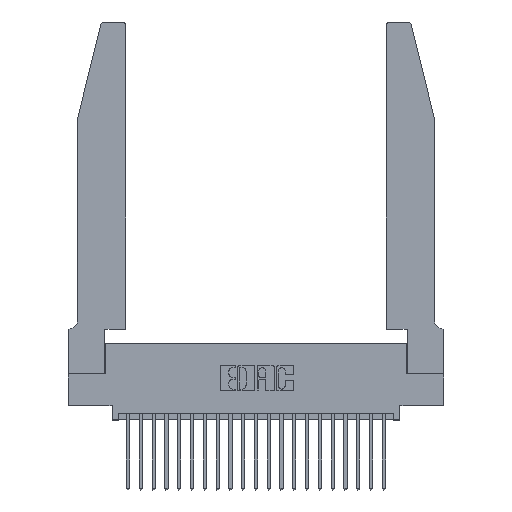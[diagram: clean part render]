
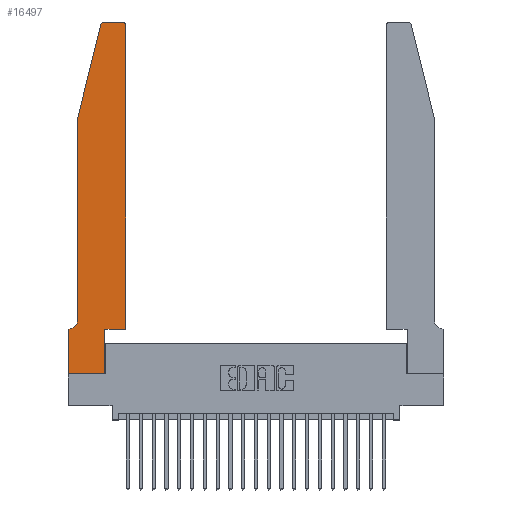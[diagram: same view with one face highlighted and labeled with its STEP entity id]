
A CAD part, top view. The second image highlights one B-rep face of the part: STEP entity #16497.
In plain terms, the highlighted planar face has unit normal (0, 0, 1).
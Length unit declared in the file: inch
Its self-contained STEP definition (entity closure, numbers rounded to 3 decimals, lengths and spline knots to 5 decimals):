
#417 = CIRCLE ( 'NONE', #15618, 0.07 ) ;
#516 = DIRECTION ( 'NONE',  ( 0., -1., 0. ) ) ;
#763 = ORIENTED_EDGE ( 'NONE', *, *, #9248, .T. ) ;
#764 = VECTOR ( 'NONE', #19577, 39.37008 ) ;
#982 = DIRECTION ( 'NONE',  ( 0., 1., 0. ) ) ;
#1370 = DIRECTION ( 'NONE',  ( -1., 0., 0. ) ) ;
#1402 = VECTOR ( 'NONE', #516, 39.37008 ) ;
#1412 = VERTEX_POINT ( 'NONE', #19674 ) ;
#1561 = VERTEX_POINT ( 'NONE', #11043 ) ;
#1594 = VERTEX_POINT ( 'NONE', #15425 ) ;
#1689 = VERTEX_POINT ( 'NONE', #3669 ) ;
#1705 = DIRECTION ( 'NONE',  ( 0., 0., 1. ) ) ;
#1916 = CARTESIAN_POINT ( 'NONE',  ( 0.0755, 2., 0.37 ) ) ;
#2494 = DIRECTION ( 'NONE',  ( 0., -1., 0. ) ) ;
#3249 = VERTEX_POINT ( 'NONE', #17881 ) ;
#3274 = DIRECTION ( 'NONE',  ( 0., 0., 1. ) ) ;
#3669 = CARTESIAN_POINT ( 'NONE',  ( 0.2865, 0., 0.37 ) ) ;
#3691 = VECTOR ( 'NONE', #982, 39.37008 ) ;
#3705 = VERTEX_POINT ( 'NONE', #4144 ) ;
#4137 = CARTESIAN_POINT ( 'NONE',  ( 0.2865, 0.35, 0.37 ) ) ;
#4144 = CARTESIAN_POINT ( 'NONE',  ( 0.284, 2.75, 0.37 ) ) ;
#4436 = AXIS2_PLACEMENT_3D ( 'NONE', #14583, #3274, #16380 ) ;
#4560 = CARTESIAN_POINT ( 'NONE',  ( 0.4205, 2.72, 0.37 ) ) ;
#4660 = CIRCLE ( 'NONE', #8988, 0.03 ) ;
#4784 = CARTESIAN_POINT ( 'NONE',  ( 0.4505, 0.35, 0.37 ) ) ;
#4839 = ORIENTED_EDGE ( 'NONE', *, *, #18056, .T. ) ;
#5339 = CARTESIAN_POINT ( 'NONE',  ( 0.2605, 2.75, 0.37 ) ) ;
#5398 = CARTESIAN_POINT ( 'NONE',  ( 0., 0.35, 0.37 ) ) ;
#5412 = EDGE_CURVE ( 'NONE', #1689, #17257, #23343, .T. ) ;
#5982 = CARTESIAN_POINT ( 'NONE',  ( 0.0755, 0.42, 0.37 ) ) ;
#6027 = LINE ( 'NONE', #19297, #1402 ) ;
#6496 = DIRECTION ( 'NONE',  ( 1., 0., 0. ) ) ;
#6662 = ORIENTED_EDGE ( 'NONE', *, *, #22767, .T. ) ;
#7354 = CARTESIAN_POINT ( 'NONE',  ( 0.25487, 2.72718, 0.37 ) ) ;
#8195 = VECTOR ( 'NONE', #2494, 39.37008 ) ;
#8217 = EDGE_CURVE ( 'NONE', #1594, #16972, #14595, .T. ) ;
#8499 = ORIENTED_EDGE ( 'NONE', *, *, #14826, .T. ) ;
#8736 = VECTOR ( 'NONE', #1370, 39.37008 ) ;
#8988 = AXIS2_PLACEMENT_3D ( 'NONE', #4560, #17552, #6496 ) ;
#9087 = VECTOR ( 'NONE', #19044, 39.37008 ) ;
#9248 = EDGE_CURVE ( 'NONE', #17257, #3249, #18185, .T. ) ;
#9323 = LINE ( 'NONE', #5339, #8736 ) ;
#9379 = PLANE ( 'NONE',  #18551 ) ;
#9465 = ORIENTED_EDGE ( 'NONE', *, *, #9613, .T. ) ;
#9613 = EDGE_CURVE ( 'NONE', #20555, #19728, #10246, .T. ) ;
#9789 = DIRECTION ( 'NONE',  ( 1., 0., 0. ) ) ;
#10006 = CARTESIAN_POINT ( 'NONE',  ( 0.4505, 0.35, 0.37 ) ) ;
#10242 = CARTESIAN_POINT ( 'NONE',  ( 0.0755, 0.35, 0.37 ) ) ;
#10246 = LINE ( 'NONE', #21478, #24086 ) ;
#10759 = ORIENTED_EDGE ( 'NONE', *, *, #22531, .T. ) ;
#11043 = CARTESIAN_POINT ( 'NONE',  ( 0., 0., 0.37 ) ) ;
#11583 = CARTESIAN_POINT ( 'NONE',  ( 0.0055, 0.42, 0.37 ) ) ;
#12852 = FACE_OUTER_BOUND ( 'NONE', #15964, .T. ) ;
#13400 = DIRECTION ( 'NONE',  ( -1., 0., 0. ) ) ;
#13519 = CIRCLE ( 'NONE', #4436, 0.03 ) ;
#13804 = LINE ( 'NONE', #22463, #22829 ) ;
#13898 = EDGE_CURVE ( 'NONE', #3705, #20555, #13519, .T. ) ;
#14163 = DIRECTION ( 'NONE',  ( -0.239, -0.971, 0. ) ) ;
#14305 = ORIENTED_EDGE ( 'NONE', *, *, #5412, .T. ) ;
#14439 = ORIENTED_EDGE ( 'NONE', *, *, #8217, .T. ) ;
#14583 = CARTESIAN_POINT ( 'NONE',  ( 0.284, 2.72, 0.37 ) ) ;
#14595 = LINE ( 'NONE', #10242, #18795 ) ;
#14826 = EDGE_CURVE ( 'NONE', #1561, #1689, #13804, .T. ) ;
#14987 = DIRECTION ( 'NONE',  ( 1., 0., 0. ) ) ;
#15004 = EDGE_CURVE ( 'NONE', #19260, #1412, #4660, .T. ) ;
#15425 = CARTESIAN_POINT ( 'NONE',  ( 0.0055, 0.35, 0.37 ) ) ;
#15618 = AXIS2_PLACEMENT_3D ( 'NONE', #11583, #24194, #13400 ) ;
#15662 = CARTESIAN_POINT ( 'NONE',  ( 0.0755, 2., 0.37 ) ) ;
#15964 = EDGE_LOOP ( 'NONE', ( #4839, #18428, #9465, #24225, #10759, #14439, #6662, #8499, #14305, #763, #19137, #20907 ) ) ;
#16349 = CARTESIAN_POINT ( 'NONE',  ( 0.4505, 2.72, 0.37 ) ) ;
#16380 = DIRECTION ( 'NONE',  ( 1., 0., 0. ) ) ;
#16491 = LINE ( 'NONE', #4784, #764 ) ;
#16497 = ADVANCED_FACE ( 'NONE', ( #12852 ), #9379, .T. ) ;
#16740 = EDGE_CURVE ( 'NONE', #19728, #21353, #21589, .T. ) ;
#16972 = VERTEX_POINT ( 'NONE', #5398 ) ;
#17257 = VERTEX_POINT ( 'NONE', #4137 ) ;
#17495 = EDGE_CURVE ( 'NONE', #3249, #19260, #16491, .T. ) ;
#17552 = DIRECTION ( 'NONE',  ( 0., 0., 1. ) ) ;
#17881 = CARTESIAN_POINT ( 'NONE',  ( 0.4505, 0.35, 0.37 ) ) ;
#18056 = EDGE_CURVE ( 'NONE', #1412, #3705, #9323, .T. ) ;
#18185 = LINE ( 'NONE', #10006, #9087 ) ;
#18428 = ORIENTED_EDGE ( 'NONE', *, *, #13898, .T. ) ;
#18551 = AXIS2_PLACEMENT_3D ( 'NONE', #22155, #1705, #14987 ) ;
#18795 = VECTOR ( 'NONE', #22966, 39.37008 ) ;
#19044 = DIRECTION ( 'NONE',  ( 1., 0., 0. ) ) ;
#19137 = ORIENTED_EDGE ( 'NONE', *, *, #17495, .T. ) ;
#19260 = VERTEX_POINT ( 'NONE', #16349 ) ;
#19297 = CARTESIAN_POINT ( 'NONE',  ( 0., 0., 0.37 ) ) ;
#19577 = DIRECTION ( 'NONE',  ( 0., 1., 0. ) ) ;
#19674 = CARTESIAN_POINT ( 'NONE',  ( 0.4205, 2.75, 0.37 ) ) ;
#19728 = VERTEX_POINT ( 'NONE', #1916 ) ;
#20555 = VERTEX_POINT ( 'NONE', #7354 ) ;
#20907 = ORIENTED_EDGE ( 'NONE', *, *, #15004, .T. ) ;
#21353 = VERTEX_POINT ( 'NONE', #5982 ) ;
#21478 = CARTESIAN_POINT ( 'NONE',  ( 0.0755, 2., 0.37 ) ) ;
#21573 = CARTESIAN_POINT ( 'NONE',  ( 0.2865, 0.35, 0.37 ) ) ;
#21589 = LINE ( 'NONE', #15662, #8195 ) ;
#22155 = CARTESIAN_POINT ( 'NONE',  ( 0., 0.35, 0.37 ) ) ;
#22463 = CARTESIAN_POINT ( 'NONE',  ( 0., 0., 0.37 ) ) ;
#22531 = EDGE_CURVE ( 'NONE', #21353, #1594, #417, .T. ) ;
#22767 = EDGE_CURVE ( 'NONE', #16972, #1561, #6027, .T. ) ;
#22829 = VECTOR ( 'NONE', #9789, 39.37008 ) ;
#22966 = DIRECTION ( 'NONE',  ( -1., 0., 0. ) ) ;
#23343 = LINE ( 'NONE', #21573, #3691 ) ;
#24086 = VECTOR ( 'NONE', #14163, 39.37008 ) ;
#24194 = DIRECTION ( 'NONE',  ( 0., 0., -1. ) ) ;
#24225 = ORIENTED_EDGE ( 'NONE', *, *, #16740, .T. ) ;
